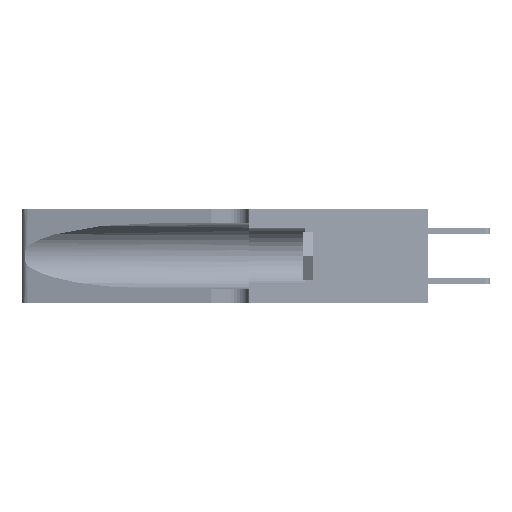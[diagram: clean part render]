
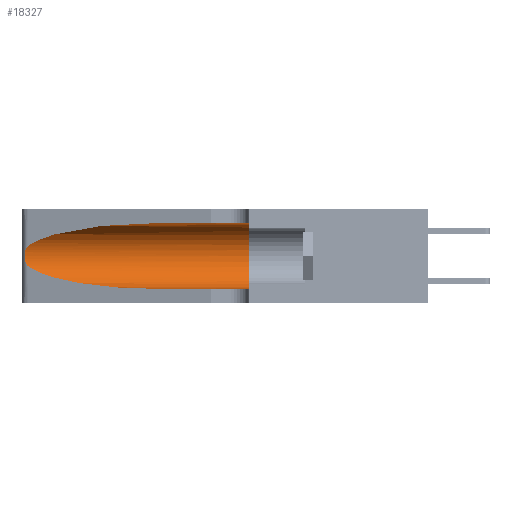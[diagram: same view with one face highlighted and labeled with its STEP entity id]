
A CAD part, left-side view. The second image highlights one B-rep face of the part: STEP entity #18327.
In plain terms, the highlighted cylindrical face has radius 3.308 mm (diameter 6.617 mm), a partial arc.
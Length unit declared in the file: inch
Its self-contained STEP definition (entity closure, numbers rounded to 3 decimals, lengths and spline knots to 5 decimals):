
#418 = CARTESIAN_POINT ( 'NONE',  ( 0.25487, 1.22718, 0.14631 ) ) ;
#1223 = B_SPLINE_CURVE_WITH_KNOTS ( 'NONE', 3,
 ( #31858, #25755, #19293, #35381, #38117, #31710, #25886, #16275, #31995, #16675, #19704, #38514, #22609, #418 ),
 .UNSPECIFIED., .F., .F.,
 ( 4, 2, 2, 2, 2, 2, 4 ),
 ( 0., 0.00027, 0.00053, 0.00107, 0.0016, 0.00187, 0.00214 ),
 .UNSPECIFIED. ) ;
#1817 = VECTOR ( 'NONE', #38160, 39.37008 ) ;
#2183 = DIRECTION ( 'NONE',  ( 0., 1., 0. ) ) ;
#2542 = EDGE_CURVE ( 'NONE', #15303, #30938, #30060, .T. ) ;
#2812 = CARTESIAN_POINT ( 'NONE',  ( 0.25487, 1.22718, 0.22369 ) ) ;
#3007 = CARTESIAN_POINT ( 'NONE',  ( 0.18966, 0.96281, 0.31525 ) ) ;
#3387 = CARTESIAN_POINT ( 'NONE',  ( 0.25487, 1.22718, 0.14631 ) ) ;
#4137 = CARTESIAN_POINT ( 'NONE',  ( 0.25487, 1.22718, 0.14631 ) ) ;
#4558 = DIRECTION ( 'NONE',  ( 0., -1., 0. ) ) ;
#6016 = CYLINDRICAL_SURFACE ( 'NONE', #28781, 0.13025 ) ;
#6117 = CARTESIAN_POINT ( 'NONE',  ( 0.1305, 0.72297, 0.05475 ) ) ;
#6231 = ORIENTED_EDGE ( 'NONE', *, *, #17921, .T. ) ;
#7181 = DIRECTION ( 'NONE',  ( 0., -1., 0. ) ) ;
#9374 = CARTESIAN_POINT ( 'NONE',  ( 0.2373, 1.15595, 0.08982 ) ) ;
#10679 = CARTESIAN_POINT ( 'NONE',  ( 0.1305, 0.35, 0.31525 ) ) ;
#10713 = EDGE_CURVE ( 'NONE', #35395, #26871, #1223, .T. ) ;
#11344 = EDGE_CURVE ( 'NONE', #30938, #15643, #36728, .T. ) ;
#11352 = CARTESIAN_POINT ( 'NONE',  ( 0.1305, 0.72297, 0.05475 ) ) ;
#12719 =( BOUNDED_CURVE ( )  B_SPLINE_CURVE ( 3, ( #34274, #3007, #15532, #34530 ),
 .UNSPECIFIED., .F., .F. ) 
 B_SPLINE_CURVE_WITH_KNOTS ( ( 4, 4 ),
 ( 1.5708, 2.84003 ),
 .UNSPECIFIED. ) 
 CURVE ( )  GEOMETRIC_REPRESENTATION_ITEM ( )  RATIONAL_B_SPLINE_CURVE ( ( 1., 0.87, 0.87, 1. ) ) 
 REPRESENTATION_ITEM ( '' )  );
#14972 = CARTESIAN_POINT ( 'NONE',  ( 0.1305, 0.35, 0.185 ) ) ;
#15303 = VERTEX_POINT ( 'NONE', #32711 ) ;
#15532 = CARTESIAN_POINT ( 'NONE',  ( 0.2373, 1.15595, 0.28018 ) ) ;
#15643 = VERTEX_POINT ( 'NONE', #18396 ) ;
#16184 = CARTESIAN_POINT ( 'NONE',  ( 0.1305, 1.61858, 0.05475 ) ) ;
#16275 = CARTESIAN_POINT ( 'NONE',  ( 0.26075, 1.23896, 0.178 ) ) ;
#16283 = AXIS2_PLACEMENT_3D ( 'NONE', #14972, #2183, #24053 ) ;
#16675 = CARTESIAN_POINT ( 'NONE',  ( 0.25856, 1.23593, 0.16098 ) ) ;
#17921 = EDGE_CURVE ( 'NONE', #15303, #35395, #12719, .T. ) ;
#18327 = ADVANCED_FACE ( 'NONE', ( #33903 ), #6016, .F. ) ;
#18396 = CARTESIAN_POINT ( 'NONE',  ( 0.1305, 0.35, 0.05475 ) ) ;
#18859 = ORIENTED_EDGE ( 'NONE', *, *, #39473, .T. ) ;
#19081 = CARTESIAN_POINT ( 'NONE',  ( 0.18966, 0.96281, 0.05475 ) ) ;
#19293 = CARTESIAN_POINT ( 'NONE',  ( 0.25639, 1.23184, 0.21858 ) ) ;
#19704 = CARTESIAN_POINT ( 'NONE',  ( 0.25789, 1.23486, 0.15765 ) ) ;
#22609 = CARTESIAN_POINT ( 'NONE',  ( 0.25555, 1.22993, 0.14849 ) ) ;
#23444 = CARTESIAN_POINT ( 'NONE',  ( 0.1305, 1.61858, 0.185 ) ) ;
#24053 = DIRECTION ( 'NONE',  ( 0., 0., 1. ) ) ;
#24064 = ORIENTED_EDGE ( 'NONE', *, *, #2542, .F. ) ;
#24719 = EDGE_LOOP ( 'NONE', ( #6231, #33617, #33911, #18859, #28517, #24064 ) ) ;
#25755 = CARTESIAN_POINT ( 'NONE',  ( 0.25555, 1.22994, 0.2215 ) ) ;
#25783 = VERTEX_POINT ( 'NONE', #11352 ) ;
#25886 = CARTESIAN_POINT ( 'NONE',  ( 0.26075, 1.23896, 0.19203 ) ) ;
#26149 = EDGE_CURVE ( 'NONE', #26871, #25783, #35008, .T. ) ;
#26871 = VERTEX_POINT ( 'NONE', #4137 ) ;
#27646 = VECTOR ( 'NONE', #7181, 39.37008 ) ;
#28517 = ORIENTED_EDGE ( 'NONE', *, *, #11344, .F. ) ;
#28781 = AXIS2_PLACEMENT_3D ( 'NONE', #23444, #4558, #32841 ) ;
#30060 = LINE ( 'NONE', #35044, #27646 ) ;
#30615 = LINE ( 'NONE', #16184, #1817 ) ;
#30938 = VERTEX_POINT ( 'NONE', #10679 ) ;
#31710 = CARTESIAN_POINT ( 'NONE',  ( 0.26018, 1.23835, 0.19895 ) ) ;
#31858 = CARTESIAN_POINT ( 'NONE',  ( 0.25487, 1.22718, 0.22369 ) ) ;
#31995 = CARTESIAN_POINT ( 'NONE',  ( 0.26017, 1.23833, 0.17102 ) ) ;
#32711 = CARTESIAN_POINT ( 'NONE',  ( 0.1305, 0.72297, 0.31525 ) ) ;
#32841 = DIRECTION ( 'NONE',  ( 0., 0., -1. ) ) ;
#33617 = ORIENTED_EDGE ( 'NONE', *, *, #10713, .T. ) ;
#33903 = FACE_OUTER_BOUND ( 'NONE', #24719, .T. ) ;
#33911 = ORIENTED_EDGE ( 'NONE', *, *, #26149, .T. ) ;
#34274 = CARTESIAN_POINT ( 'NONE',  ( 0.1305, 0.72297, 0.31525 ) ) ;
#34530 = CARTESIAN_POINT ( 'NONE',  ( 0.25487, 1.22718, 0.22369 ) ) ;
#35008 =( BOUNDED_CURVE ( )  B_SPLINE_CURVE ( 3, ( #3387, #9374, #19081, #6117 ),
 .UNSPECIFIED., .F., .F. ) 
 B_SPLINE_CURVE_WITH_KNOTS ( ( 4, 4 ),
 ( 3.44316, 4.71239 ),
 .UNSPECIFIED. ) 
 CURVE ( )  GEOMETRIC_REPRESENTATION_ITEM ( )  RATIONAL_B_SPLINE_CURVE ( ( 1., 0.87, 0.87, 1. ) ) 
 REPRESENTATION_ITEM ( '' )  );
#35044 = CARTESIAN_POINT ( 'NONE',  ( 0.1305, 1.61858, 0.31525 ) ) ;
#35381 = CARTESIAN_POINT ( 'NONE',  ( 0.25787, 1.23484, 0.2124 ) ) ;
#35395 = VERTEX_POINT ( 'NONE', #2812 ) ;
#36728 = CIRCLE ( 'NONE', #16283, 0.13025 ) ;
#38117 = CARTESIAN_POINT ( 'NONE',  ( 0.25854, 1.2359, 0.20912 ) ) ;
#38160 = DIRECTION ( 'NONE',  ( 0., -1., 0. ) ) ;
#38514 = CARTESIAN_POINT ( 'NONE',  ( 0.25639, 1.23186, 0.15144 ) ) ;
#39473 = EDGE_CURVE ( 'NONE', #25783, #15643, #30615, .T. ) ;
